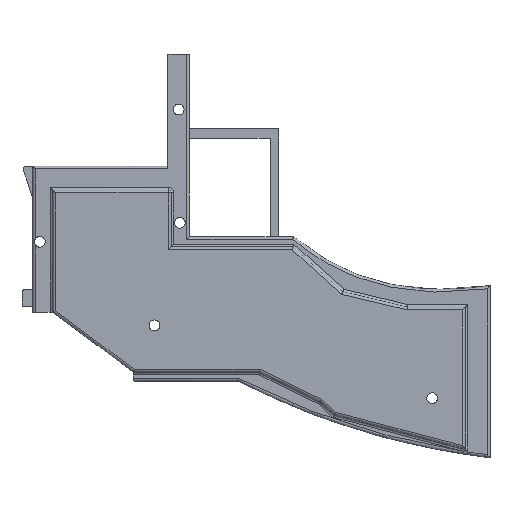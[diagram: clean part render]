
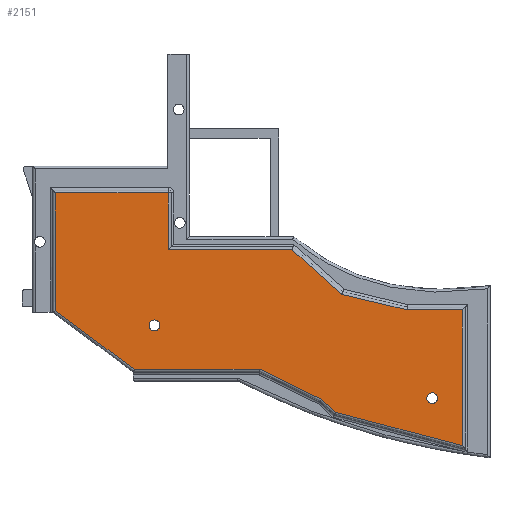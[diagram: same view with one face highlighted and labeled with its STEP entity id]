
A CAD part, left-side view. The second image highlights one B-rep face of the part: STEP entity #2151.
In plain terms, the highlighted planar face has unit normal (-1, 0, 0).
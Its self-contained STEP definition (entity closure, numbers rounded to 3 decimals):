
#47 = CARTESIAN_POINT ( 'NONE',  ( -3., -101.204, -97.278 ) ) ;
#56 = CARTESIAN_POINT ( 'NONE',  ( -3., 49.693, -97.619 ) ) ;
#59 = CARTESIAN_POINT ( 'NONE',  ( -3., 20.464, -119.36 ) ) ;
#62 = CARTESIAN_POINT ( 'NONE',  ( -3., -26.225, -119.36 ) ) ;
#65 = CARTESIAN_POINT ( 'NONE',  ( -3., -48.884, -130.481 ) ) ;
#68 = CARTESIAN_POINT ( 'NONE',  ( -3., -54.185, -135.238 ) ) ;
#71 = CARTESIAN_POINT ( 'NONE',  ( -3., -101.204, -147.596 ) ) ;
#83 = CARTESIAN_POINT ( 'NONE',  ( -3., 7.798, -74.919 ) ) ;
#84 = CARTESIAN_POINT ( 'NONE',  ( -3., 7.798, -53.871 ) ) ;
#94 = CARTESIAN_POINT ( 'NONE',  ( -3., 49.693, -53.871 ) ) ;
#119 = CARTESIAN_POINT ( 'NONE',  ( -3., 13., -101. ) ) ;
#120 = CARTESIAN_POINT ( 'NONE',  ( -3., 13., -105. ) ) ;
#126 = CARTESIAN_POINT ( 'NONE',  ( -3., -90., -132. ) ) ;
#137 = CARTESIAN_POINT ( 'NONE',  ( -3., -90., -128. ) ) ;
#586 = CARTESIAN_POINT ( 'NONE',  ( -3., -80.691, -97.278 ) ) ;
#630 = CIRCLE ( 'NONE', #6542, 2. ) ;
#727 = CIRCLE ( 'NONE', #1523, 2. ) ;
#889 = VERTEX_POINT ( 'NONE', #137 ) ;
#892 = VERTEX_POINT ( 'NONE', #126 ) ;
#898 = VERTEX_POINT ( 'NONE', #120 ) ;
#899 = VERTEX_POINT ( 'NONE', #119 ) ;
#1127 = EDGE_LOOP ( 'NONE', ( #3546, #3547, #3548, #3549, #3550, #3551, #3552, #3553, #3554, #3555, #3556, #3557, #3558 ) ) ;
#1134 = EDGE_LOOP ( 'NONE', ( #3561, #3562 ) ) ;
#1135 = EDGE_LOOP ( 'NONE', ( #3559, #3560 ) ) ;
#1400 = CARTESIAN_POINT ( 'NONE',  ( -3., -56.435, -91.492 ) ) ;
#1403 = CARTESIAN_POINT ( 'NONE',  ( -3., -37.965, -74.919 ) ) ;
#1523 = AXIS2_PLACEMENT_3D ( 'NONE', #5398, #5399, #5400 ) ;
#1905 = DIRECTION ( 'NONE',  ( 0., 0., -1. ) ) ;
#1910 = PLANE ( 'NONE',  #6443 ) ;
#1912 = CARTESIAN_POINT ( 'NONE',  ( -3., 0., 0. ) ) ;
#1915 = DIRECTION ( 'NONE',  ( 1., 0., 0. ) ) ;
#2151 = ADVANCED_FACE ( 'NONE', ( #7065, #7067, #7064 ), #1910, .F. ) ;
#2308 = VERTEX_POINT ( 'NONE', #94 ) ;
#2311 = VERTEX_POINT ( 'NONE', #84 ) ;
#2313 = VERTEX_POINT ( 'NONE', #83 ) ;
#2318 = VERTEX_POINT ( 'NONE', #71 ) ;
#2319 = VERTEX_POINT ( 'NONE', #68 ) ;
#2320 = VERTEX_POINT ( 'NONE', #65 ) ;
#2321 = VERTEX_POINT ( 'NONE', #62 ) ;
#2322 = VERTEX_POINT ( 'NONE', #59 ) ;
#2323 = VERTEX_POINT ( 'NONE', #56 ) ;
#2325 = VERTEX_POINT ( 'NONE', #47 ) ;
#2634 = VERTEX_POINT ( 'NONE', #1403 ) ;
#2636 = VERTEX_POINT ( 'NONE', #586 ) ;
#2637 = VERTEX_POINT ( 'NONE', #1400 ) ;
#3546 = ORIENTED_EDGE ( 'NONE', *, *, #6214, .T. ) ;
#3547 = ORIENTED_EDGE ( 'NONE', *, *, #6215, .T. ) ;
#3548 = ORIENTED_EDGE ( 'NONE', *, *, #6216, .T. ) ;
#3549 = ORIENTED_EDGE ( 'NONE', *, *, #6217, .T. ) ;
#3550 = ORIENTED_EDGE ( 'NONE', *, *, #6218, .T. ) ;
#3551 = ORIENTED_EDGE ( 'NONE', *, *, #6219, .T. ) ;
#3552 = ORIENTED_EDGE ( 'NONE', *, *, #6220, .T. ) ;
#3553 = ORIENTED_EDGE ( 'NONE', *, *, #6221, .T. ) ;
#3554 = ORIENTED_EDGE ( 'NONE', *, *, #6222, .T. ) ;
#3555 = ORIENTED_EDGE ( 'NONE', *, *, #6223, .T. ) ;
#3556 = ORIENTED_EDGE ( 'NONE', *, *, #6224, .T. ) ;
#3557 = ORIENTED_EDGE ( 'NONE', *, *, #6225, .T. ) ;
#3558 = ORIENTED_EDGE ( 'NONE', *, *, #6226, .T. ) ;
#3559 = ORIENTED_EDGE ( 'NONE', *, *, #6227, .T. ) ;
#3560 = ORIENTED_EDGE ( 'NONE', *, *, #6290, .T. ) ;
#3561 = ORIENTED_EDGE ( 'NONE', *, *, #6228, .F. ) ;
#3562 = ORIENTED_EDGE ( 'NONE', *, *, #6354, .F. ) ;
#5049 = CARTESIAN_POINT ( 'NONE',  ( -3., 0., -53.871 ) ) ;
#5052 = CARTESIAN_POINT ( 'NONE',  ( -3., 7.798, 0. ) ) ;
#5054 = DIRECTION ( 'NONE',  ( 0., 0., 1. ) ) ;
#5055 = DIRECTION ( 'NONE',  ( 0., 1., 0. ) ) ;
#5056 = CARTESIAN_POINT ( 'NONE',  ( -3., 49.693, 0. ) ) ;
#5057 = DIRECTION ( 'NONE',  ( 0., 0., -1. ) ) ;
#5058 = CARTESIAN_POINT ( 'NONE',  ( -3., 64.447, -86.645 ) ) ;
#5059 = DIRECTION ( 'NONE',  ( 0., -0.802, -0.597 ) ) ;
#5060 = CARTESIAN_POINT ( 'NONE',  ( -3., 0., -119.36 ) ) ;
#5061 = DIRECTION ( 'NONE',  ( 0., -1., 0. ) ) ;
#5062 = CARTESIAN_POINT ( 'NONE',  ( -3., 42.119, -85.818 ) ) ;
#5063 = DIRECTION ( 'NONE',  ( 0., -0.898, -0.441 ) ) ;
#5064 = CARTESIAN_POINT ( 'NONE',  ( -3., 43.055, -47.982 ) ) ;
#5065 = DIRECTION ( 'NONE',  ( 0., -0.744, -0.668 ) ) ;
#5066 = CARTESIAN_POINT ( 'NONE',  ( -3., 29.747, -113.178 ) ) ;
#5067 = DIRECTION ( 'NONE',  ( 0., -0.967, -0.254 ) ) ;
#5068 = CARTESIAN_POINT ( 'NONE',  ( -3., -101.204, 0. ) ) ;
#5069 = DIRECTION ( 'NONE',  ( 0., 0., 1. ) ) ;
#5070 = CARTESIAN_POINT ( 'NONE',  ( -3., 0., -97.278 ) ) ;
#5071 = DIRECTION ( 'NONE',  ( 0., 1., 0. ) ) ;
#5072 = CARTESIAN_POINT ( 'NONE',  ( -3., 17.61, -73.832 ) ) ;
#5073 = DIRECTION ( 'NONE',  ( 0., 0.973, 0.232 ) ) ;
#5074 = CARTESIAN_POINT ( 'NONE',  ( -3., 20.307, -22.63 ) ) ;
#5075 = DIRECTION ( 'NONE',  ( 0., 0.744, 0.668 ) ) ;
#5076 = CARTESIAN_POINT ( 'NONE',  ( -3., 0., -74.919 ) ) ;
#5077 = DIRECTION ( 'NONE',  ( 0., 1., 0. ) ) ;
#5079 = CARTESIAN_POINT ( 'NONE',  ( -3., -90., -130. ) ) ;
#5080 = DIRECTION ( 'NONE',  ( 1., 0., 0. ) ) ;
#5081 = DIRECTION ( 'NONE',  ( 0., 0., -1. ) ) ;
#5082 = CARTESIAN_POINT ( 'NONE',  ( -3., 13., -103. ) ) ;
#5083 = DIRECTION ( 'NONE',  ( -1., 0., 0. ) ) ;
#5084 = DIRECTION ( 'NONE',  ( 0., 0., -1. ) ) ;
#5215 = CARTESIAN_POINT ( 'NONE',  ( -3., -90., -130. ) ) ;
#5216 = DIRECTION ( 'NONE',  ( 1., 0., 0. ) ) ;
#5217 = DIRECTION ( 'NONE',  ( 0., 0., -1. ) ) ;
#5398 = CARTESIAN_POINT ( 'NONE',  ( -3., 13., -103. ) ) ;
#5399 = DIRECTION ( 'NONE',  ( -1., 0., 0. ) ) ;
#5400 = DIRECTION ( 'NONE',  ( 0., 0., -1. ) ) ;
#5719 = LINE ( 'NONE', #5049, #5726 ) ;
#5721 = LINE ( 'NONE', #5052, #5724 ) ;
#5723 = CIRCLE ( 'NONE', #6535, 2. ) ;
#5724 = VECTOR ( 'NONE', #5054, 1000. ) ;
#5725 = LINE ( 'NONE', #5056, #5728 ) ;
#5726 = VECTOR ( 'NONE', #5055, 1000. ) ;
#5727 = LINE ( 'NONE', #5058, #5730 ) ;
#5728 = VECTOR ( 'NONE', #5057, 1000. ) ;
#5729 = LINE ( 'NONE', #5060, #5732 ) ;
#5730 = VECTOR ( 'NONE', #5059, 1000. ) ;
#5731 = LINE ( 'NONE', #5062, #5734 ) ;
#5732 = VECTOR ( 'NONE', #5061, 1000. ) ;
#5733 = LINE ( 'NONE', #5064, #5736 ) ;
#5734 = VECTOR ( 'NONE', #5063, 1000. ) ;
#5735 = LINE ( 'NONE', #5066, #5738 ) ;
#5736 = VECTOR ( 'NONE', #5065, 1000. ) ;
#5737 = LINE ( 'NONE', #5068, #5740 ) ;
#5738 = VECTOR ( 'NONE', #5067, 1000. ) ;
#5739 = LINE ( 'NONE', #5070, #5742 ) ;
#5740 = VECTOR ( 'NONE', #5069, 1000. ) ;
#5741 = LINE ( 'NONE', #5072, #5744 ) ;
#5742 = VECTOR ( 'NONE', #5071, 1000. ) ;
#5743 = LINE ( 'NONE', #5074, #5746 ) ;
#5744 = VECTOR ( 'NONE', #5073, 1000. ) ;
#5745 = LINE ( 'NONE', #5076, #5748 ) ;
#5746 = VECTOR ( 'NONE', #5075, 1000. ) ;
#5747 = CIRCLE ( 'NONE', #6534, 2. ) ;
#5748 = VECTOR ( 'NONE', #5077, 1000. ) ;
#6214 = EDGE_CURVE ( 'NONE', #2313, #2311, #5721, .T. ) ;
#6215 = EDGE_CURVE ( 'NONE', #2311, #2308, #5719, .T. ) ;
#6216 = EDGE_CURVE ( 'NONE', #2308, #2323, #5725, .T. ) ;
#6217 = EDGE_CURVE ( 'NONE', #2323, #2322, #5727, .T. ) ;
#6218 = EDGE_CURVE ( 'NONE', #2322, #2321, #5729, .T. ) ;
#6219 = EDGE_CURVE ( 'NONE', #2321, #2320, #5731, .T. ) ;
#6220 = EDGE_CURVE ( 'NONE', #2320, #2319, #5733, .T. ) ;
#6221 = EDGE_CURVE ( 'NONE', #2319, #2318, #5735, .T. ) ;
#6222 = EDGE_CURVE ( 'NONE', #2318, #2325, #5737, .T. ) ;
#6223 = EDGE_CURVE ( 'NONE', #2325, #2636, #5739, .T. ) ;
#6224 = EDGE_CURVE ( 'NONE', #2636, #2637, #5741, .T. ) ;
#6225 = EDGE_CURVE ( 'NONE', #2637, #2634, #5743, .T. ) ;
#6226 = EDGE_CURVE ( 'NONE', #2634, #2313, #5745, .T. ) ;
#6227 = EDGE_CURVE ( 'NONE', #892, #889, #5747, .T. ) ;
#6228 = EDGE_CURVE ( 'NONE', #899, #898, #5723, .T. ) ;
#6290 = EDGE_CURVE ( 'NONE', #889, #892, #630, .T. ) ;
#6354 = EDGE_CURVE ( 'NONE', #898, #899, #727, .T. ) ;
#6443 = AXIS2_PLACEMENT_3D ( 'NONE', #1912, #1915, #1905 ) ;
#6534 = AXIS2_PLACEMENT_3D ( 'NONE', #5079, #5080, #5081 ) ;
#6535 = AXIS2_PLACEMENT_3D ( 'NONE', #5082, #5083, #5084 ) ;
#6542 = AXIS2_PLACEMENT_3D ( 'NONE', #5215, #5216, #5217 ) ;
#7064 = FACE_BOUND ( 'NONE', #1134, .T. ) ;
#7065 = FACE_OUTER_BOUND ( 'NONE', #1127, .T. ) ;
#7067 = FACE_BOUND ( 'NONE', #1135, .T. ) ;
